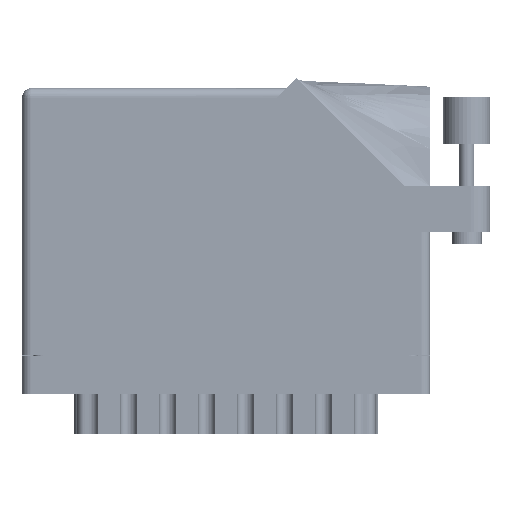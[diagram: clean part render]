
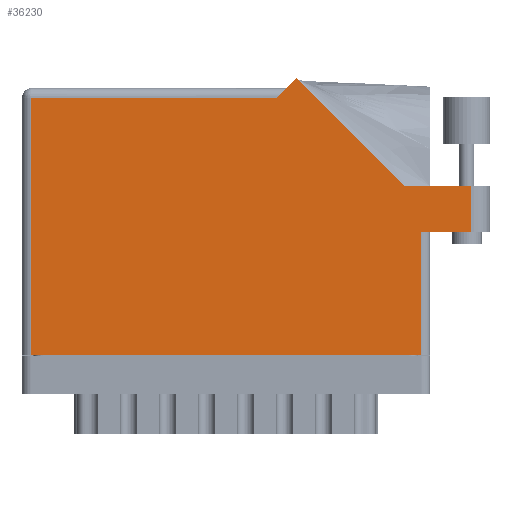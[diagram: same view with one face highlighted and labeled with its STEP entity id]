
A CAD part, front view. The second image highlights one B-rep face of the part: STEP entity #36230.
In plain terms, the highlighted face is planar.
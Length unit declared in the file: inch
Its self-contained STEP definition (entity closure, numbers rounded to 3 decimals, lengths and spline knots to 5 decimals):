
#48 = LINE ( 'NONE', #44481, #39802 ) ;
#978 = LINE ( 'NONE', #69430, #24111 ) ;
#1729 = DIRECTION ( 'NONE',  ( -1., 0., 0. ) ) ;
#2908 = EDGE_CURVE ( 'NONE', #75498, #55894, #48, .T. ) ;
#2972 = CARTESIAN_POINT ( 'NONE',  ( 2.656, 0.815, 0. ) ) ;
#6384 = ORIENTED_EDGE ( 'NONE', *, *, #15075, .T. ) ;
#7137 = VERTEX_POINT ( 'NONE', #53922 ) ;
#7170 = CARTESIAN_POINT ( 'NONE',  ( 2.993, 0.815, 0. ) ) ;
#7447 = CARTESIAN_POINT ( 'NONE',  ( 2.993, 1.122, 0. ) ) ;
#8458 = LINE ( 'NONE', #62077, #61169 ) ;
#8479 = VECTOR ( 'NONE', #59843, 39.37008 ) ;
#8742 = ORIENTED_EDGE ( 'NONE', *, *, #2908, .T. ) ;
#8916 = VECTOR ( 'NONE', #65490, 39.37008 ) ;
#9606 = EDGE_CURVE ( 'NONE', #53451, #49416, #64929, .T. ) ;
#12785 = CARTESIAN_POINT ( 'NONE',  ( 1.82871, 1.84571, 0. ) ) ;
#13503 = LINE ( 'NONE', #64671, #28330 ) ;
#15075 = EDGE_CURVE ( 'NONE', #7137, #23143, #13503, .T. ) ;
#15465 = LINE ( 'NONE', #25003, #44136 ) ;
#18826 = EDGE_CURVE ( 'NONE', #49416, #7137, #978, .T. ) ;
#19988 = LINE ( 'NONE', #24404, #8916 ) ;
#20032 = FACE_OUTER_BOUND ( 'NONE', #54168, .T. ) ;
#20254 = CARTESIAN_POINT ( 'NONE',  ( 0.062, 1.713, 0. ) ) ;
#20315 = ORIENTED_EDGE ( 'NONE', *, *, #18826, .T. ) ;
#20711 = AXIS2_PLACEMENT_3D ( 'NONE', #50699, #27481, #68560 ) ;
#21419 = VECTOR ( 'NONE', #74745, 39.37008 ) ;
#23143 = VERTEX_POINT ( 'NONE', #20254 ) ;
#23266 = EDGE_CURVE ( 'NONE', #23143, #69361, #8458, .T. ) ;
#24081 = CARTESIAN_POINT ( 'NONE',  ( 2.656, 0., 0. ) ) ;
#24111 = VECTOR ( 'NONE', #74817, 39.37008 ) ;
#24404 = CARTESIAN_POINT ( 'NONE',  ( 0., 0., 0. ) ) ;
#25003 = CARTESIAN_POINT ( 'NONE',  ( 3.118, 1.122, 0. ) ) ;
#27481 = DIRECTION ( 'NONE',  ( 0., 0., -1. ) ) ;
#28330 = VECTOR ( 'NONE', #58724, 39.37008 ) ;
#28445 = EDGE_CURVE ( 'NONE', #55894, #70470, #35905, .T. ) ;
#32414 = DIRECTION ( 'NONE',  ( 0., -1., 0. ) ) ;
#34554 = ORIENTED_EDGE ( 'NONE', *, *, #50545, .T. ) ;
#35046 = ORIENTED_EDGE ( 'NONE', *, *, #74346, .T. ) ;
#35905 = LINE ( 'NONE', #7447, #61702 ) ;
#36230 = ADVANCED_FACE ( 'NONE', ( #20032 ), #70366, .F. ) ;
#36969 = CARTESIAN_POINT ( 'NONE',  ( 2.993, 1.122, 0. ) ) ;
#39802 = VECTOR ( 'NONE', #62494, 39.37008 ) ;
#41883 = VERTEX_POINT ( 'NONE', #24081 ) ;
#44136 = VECTOR ( 'NONE', #1729, 39.37008 ) ;
#44481 = CARTESIAN_POINT ( 'NONE',  ( 2.718, 0.815, 0. ) ) ;
#44557 = CARTESIAN_POINT ( 'NONE',  ( 0.062, 0., 0. ) ) ;
#45193 = ORIENTED_EDGE ( 'NONE', *, *, #51110, .T. ) ;
#46232 = CARTESIAN_POINT ( 'NONE',  ( 2.55242, 1.122, 0. ) ) ;
#49416 = VERTEX_POINT ( 'NONE', #12785 ) ;
#50545 = EDGE_CURVE ( 'NONE', #70470, #53451, #15465, .T. ) ;
#50699 = CARTESIAN_POINT ( 'NONE',  ( 0., 1.775, 0. ) ) ;
#51110 = EDGE_CURVE ( 'NONE', #69361, #41883, #19988, .T. ) ;
#51932 = LINE ( 'NONE', #2972, #21419 ) ;
#53451 = VERTEX_POINT ( 'NONE', #46232 ) ;
#53922 = CARTESIAN_POINT ( 'NONE',  ( 1.696, 1.713, 0. ) ) ;
#54168 = EDGE_LOOP ( 'NONE', ( #8742, #59970, #34554, #67560, #20315, #6384, #65374, #45193, #35046 ) ) ;
#55894 = VERTEX_POINT ( 'NONE', #7170 ) ;
#58724 = DIRECTION ( 'NONE',  ( -1., 0., 0. ) ) ;
#59843 = DIRECTION ( 'NONE',  ( -0.707, 0.707, 0. ) ) ;
#59970 = ORIENTED_EDGE ( 'NONE', *, *, #28445, .T. ) ;
#61169 = VECTOR ( 'NONE', #32414, 39.37008 ) ;
#61702 = VECTOR ( 'NONE', #67140, 39.37008 ) ;
#62077 = CARTESIAN_POINT ( 'NONE',  ( 0.062, 0., 0. ) ) ;
#62494 = DIRECTION ( 'NONE',  ( 1., 0., 0. ) ) ;
#64671 = CARTESIAN_POINT ( 'NONE',  ( 0., 1.713, 0. ) ) ;
#64929 = LINE ( 'NONE', #72485, #8479 ) ;
#65374 = ORIENTED_EDGE ( 'NONE', *, *, #23266, .T. ) ;
#65490 = DIRECTION ( 'NONE',  ( 1., 0., 0. ) ) ;
#67140 = DIRECTION ( 'NONE',  ( 0., 1., 0. ) ) ;
#67560 = ORIENTED_EDGE ( 'NONE', *, *, #9606, .T. ) ;
#67771 = CARTESIAN_POINT ( 'NONE',  ( 2.656, 0.815, 0. ) ) ;
#68560 = DIRECTION ( 'NONE',  ( -1., 0., 0. ) ) ;
#69361 = VERTEX_POINT ( 'NONE', #44557 ) ;
#69430 = CARTESIAN_POINT ( 'NONE',  ( 1.758, 1.775, 0. ) ) ;
#70366 = PLANE ( 'NONE',  #20711 ) ;
#70470 = VERTEX_POINT ( 'NONE', #36969 ) ;
#72485 = CARTESIAN_POINT ( 'NONE',  ( 2.55242, 1.122, 0. ) ) ;
#74346 = EDGE_CURVE ( 'NONE', #41883, #75498, #51932, .T. ) ;
#74745 = DIRECTION ( 'NONE',  ( 0., 1., 0. ) ) ;
#74817 = DIRECTION ( 'NONE',  ( -0.707, -0.707, 0. ) ) ;
#75498 = VERTEX_POINT ( 'NONE', #67771 ) ;
